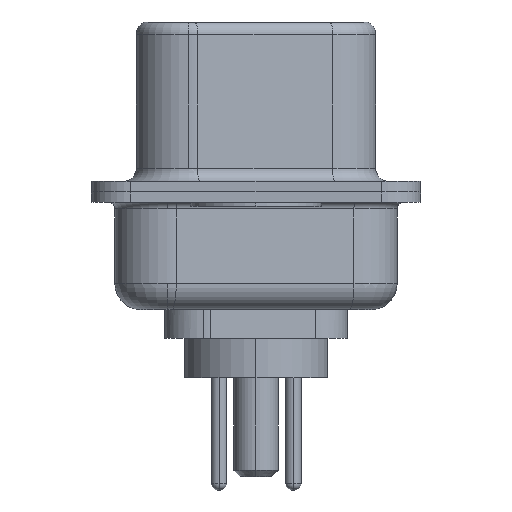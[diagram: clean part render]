
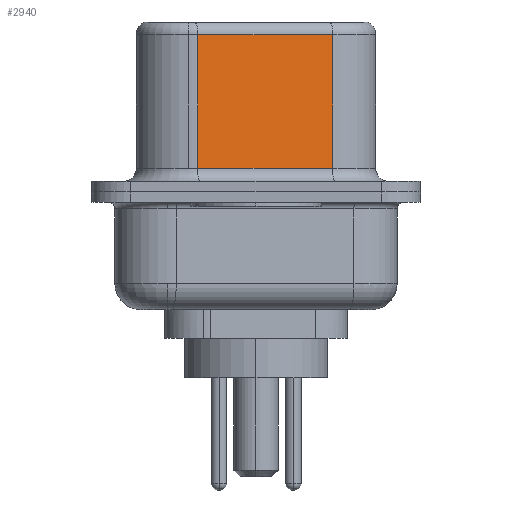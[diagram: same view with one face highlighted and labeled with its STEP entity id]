
A CAD part, left-side view. The second image highlights one B-rep face of the part: STEP entity #2940.
In plain terms, the highlighted planar face has unit normal (-0.985, -0.174, 0).
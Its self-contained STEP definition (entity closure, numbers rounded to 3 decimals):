
#167 = ORIENTED_EDGE ( 'NONE', *, *, #9472, .T. ) ;
#995 = VERTEX_POINT ( 'NONE', #6511 ) ;
#1145 = DIRECTION ( 'NONE',  ( -0.174, 0.985, 0. ) ) ;
#1158 = EDGE_CURVE ( 'NONE', #995, #12919, #6315, .T. ) ;
#1791 = DIRECTION ( 'NONE',  ( 0.985, 0.174, 0. ) ) ;
#1982 = LINE ( 'NONE', #4654, #14187 ) ;
#2239 = VECTOR ( 'NONE', #3543, 1000. ) ;
#2940 = ADVANCED_FACE ( 'NONE', ( #11712 ), #3532, .F. ) ;
#3103 = VECTOR ( 'NONE', #12931, 1000. ) ;
#3197 = DIRECTION ( 'NONE',  ( 0., 0., -1. ) ) ;
#3532 = PLANE ( 'NONE',  #14723 ) ;
#3543 = DIRECTION ( 'NONE',  ( 0., 0., -1. ) ) ;
#3575 = EDGE_CURVE ( 'NONE', #10431, #12919, #1982, .T. ) ;
#4557 = EDGE_LOOP ( 'NONE', ( #10618, #4868, #167, #15131 ) ) ;
#4654 = CARTESIAN_POINT ( 'NONE',  ( 4.585, -2.927, 0.9 ) ) ;
#4740 = CARTESIAN_POINT ( 'NONE',  ( 3.675, 2.233, 6.52 ) ) ;
#4868 = ORIENTED_EDGE ( 'NONE', *, *, #6492, .T. ) ;
#5355 = CARTESIAN_POINT ( 'NONE',  ( 4.585, -2.927, 6.52 ) ) ;
#6315 = LINE ( 'NONE', #5355, #12192 ) ;
#6492 = EDGE_CURVE ( 'NONE', #995, #12548, #12121, .T. ) ;
#6511 = CARTESIAN_POINT ( 'NONE',  ( 4.585, -2.927, 6.02 ) ) ;
#6799 = CARTESIAN_POINT ( 'NONE',  ( 4.585, -2.927, 6.52 ) ) ;
#8770 = CARTESIAN_POINT ( 'NONE',  ( 3.675, 2.233, 0.9 ) ) ;
#9472 = EDGE_CURVE ( 'NONE', #12548, #10431, #14828, .T. ) ;
#10431 = VERTEX_POINT ( 'NONE', #8770 ) ;
#10618 = ORIENTED_EDGE ( 'NONE', *, *, #1158, .F. ) ;
#11468 = CARTESIAN_POINT ( 'NONE',  ( 3.675, 2.233, 6.02 ) ) ;
#11712 = FACE_OUTER_BOUND ( 'NONE', #4557, .T. ) ;
#12121 = LINE ( 'NONE', #14906, #3103 ) ;
#12192 = VECTOR ( 'NONE', #3197, 1000. ) ;
#12548 = VERTEX_POINT ( 'NONE', #11468 ) ;
#12696 = DIRECTION ( 'NONE',  ( 0.174, -0.985, 0. ) ) ;
#12919 = VERTEX_POINT ( 'NONE', #13360 ) ;
#12931 = DIRECTION ( 'NONE',  ( -0.174, 0.985, 0. ) ) ;
#13360 = CARTESIAN_POINT ( 'NONE',  ( 4.585, -2.927, 0.9 ) ) ;
#14187 = VECTOR ( 'NONE', #12696, 1000. ) ;
#14723 = AXIS2_PLACEMENT_3D ( 'NONE', #6799, #1791, #1145 ) ;
#14828 = LINE ( 'NONE', #4740, #2239 ) ;
#14906 = CARTESIAN_POINT ( 'NONE',  ( 4.585, -2.927, 6.02 ) ) ;
#15131 = ORIENTED_EDGE ( 'NONE', *, *, #3575, .T. ) ;
